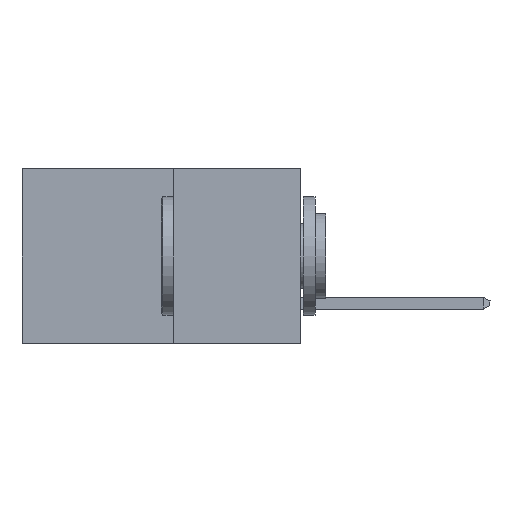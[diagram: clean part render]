
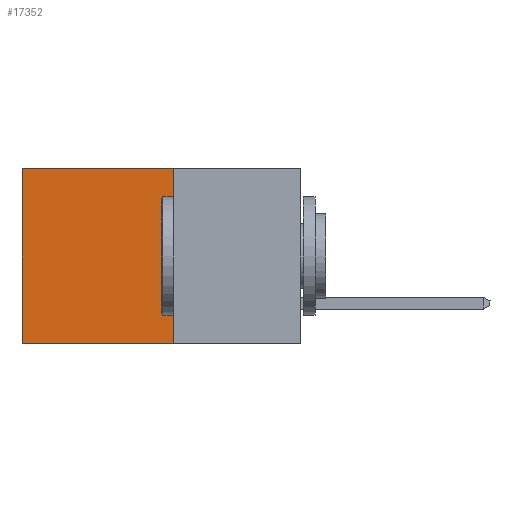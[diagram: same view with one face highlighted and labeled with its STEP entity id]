
A CAD part, left-side view. The second image highlights one B-rep face of the part: STEP entity #17352.
In plain terms, the highlighted planar face has unit normal (-1, 0, 0).
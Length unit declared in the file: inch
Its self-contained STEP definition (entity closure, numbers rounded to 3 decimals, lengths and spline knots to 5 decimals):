
#1206 = VERTEX_POINT ( 'NONE', #7345 ) ;
#1569 = CARTESIAN_POINT ( 'NONE',  ( 0.277, 0.59, -0.37 ) ) ;
#2738 = DIRECTION ( 'NONE',  ( 0., 0., -1. ) ) ;
#4542 = CARTESIAN_POINT ( 'NONE',  ( 0.277, 0.59, -0.37 ) ) ;
#5043 = VERTEX_POINT ( 'NONE', #27778 ) ;
#6679 = VECTOR ( 'NONE', #2738, 39.37008 ) ;
#7345 = CARTESIAN_POINT ( 'NONE',  ( 0.277, 0.27, 0. ) ) ;
#7373 = DIRECTION ( 'NONE',  ( 0., 1., 0. ) ) ;
#8816 = DIRECTION ( 'NONE',  ( 1., 0., 0. ) ) ;
#10072 = ORIENTED_EDGE ( 'NONE', *, *, #14732, .F. ) ;
#10228 = VECTOR ( 'NONE', #29155, 39.37008 ) ;
#11200 = PLANE ( 'NONE',  #21334 ) ;
#11434 = LINE ( 'NONE', #12019, #24046 ) ;
#11574 = EDGE_CURVE ( 'NONE', #5043, #14705, #20134, .T. ) ;
#12019 = CARTESIAN_POINT ( 'NONE',  ( 0.277, 0.27, -0.37 ) ) ;
#13685 = ORIENTED_EDGE ( 'NONE', *, *, #16327, .T. ) ;
#13715 = VECTOR ( 'NONE', #7373, 39.37008 ) ;
#14556 = DIRECTION ( 'NONE',  ( 0., 1., 0. ) ) ;
#14705 = VERTEX_POINT ( 'NONE', #1569 ) ;
#14732 = EDGE_CURVE ( 'NONE', #19547, #14705, #11434, .T. ) ;
#16290 = CARTESIAN_POINT ( 'NONE',  ( 0.277, 0.27, -0.37 ) ) ;
#16327 = EDGE_CURVE ( 'NONE', #1206, #5043, #20391, .T. ) ;
#16551 = CARTESIAN_POINT ( 'NONE',  ( 0.277, 0.27, -0.37 ) ) ;
#16846 = CARTESIAN_POINT ( 'NONE',  ( 0.277, 0.27, -0.37 ) ) ;
#16925 = LINE ( 'NONE', #16551, #10228 ) ;
#17352 = ADVANCED_FACE ( 'NONE', ( #27388 ), #11200, .F. ) ;
#19547 = VERTEX_POINT ( 'NONE', #16846 ) ;
#19975 = CARTESIAN_POINT ( 'NONE',  ( 0.277, 0.27, 0. ) ) ;
#20134 = LINE ( 'NONE', #4542, #6679 ) ;
#20391 = LINE ( 'NONE', #19975, #13715 ) ;
#21334 = AXIS2_PLACEMENT_3D ( 'NONE', #16290, #8816, #26396 ) ;
#24046 = VECTOR ( 'NONE', #14556, 39.37008 ) ;
#26396 = DIRECTION ( 'NONE',  ( 0., 0., -1. ) ) ;
#27388 = FACE_OUTER_BOUND ( 'NONE', #32575, .T. ) ;
#27778 = CARTESIAN_POINT ( 'NONE',  ( 0.277, 0.59, 0. ) ) ;
#28123 = ORIENTED_EDGE ( 'NONE', *, *, #28830, .F. ) ;
#28830 = EDGE_CURVE ( 'NONE', #1206, #19547, #16925, .T. ) ;
#29155 = DIRECTION ( 'NONE',  ( 0., 0., -1. ) ) ;
#30233 = ORIENTED_EDGE ( 'NONE', *, *, #11574, .T. ) ;
#32575 = EDGE_LOOP ( 'NONE', ( #30233, #10072, #28123, #13685 ) ) ;
